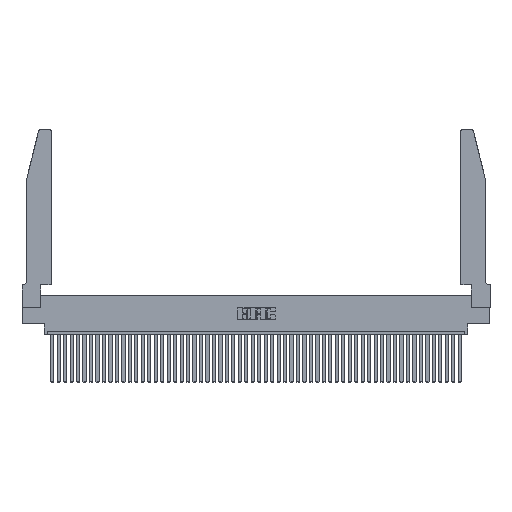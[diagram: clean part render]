
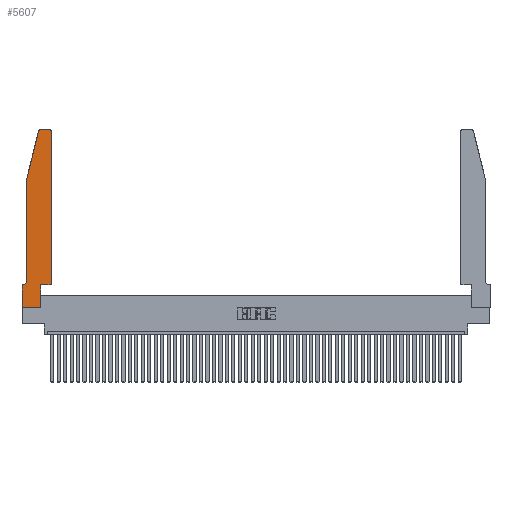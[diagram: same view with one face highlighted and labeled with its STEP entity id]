
A CAD part, top view. The second image highlights one B-rep face of the part: STEP entity #5607.
In plain terms, the highlighted planar face has unit normal (0, 0, 1).
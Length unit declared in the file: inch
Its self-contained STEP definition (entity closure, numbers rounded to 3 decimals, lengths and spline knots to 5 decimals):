
#176 = LINE ( 'NONE', #29525, #39927 ) ;
#770 = EDGE_CURVE ( 'NONE', #45909, #34590, #813, .T. ) ;
#813 = CIRCLE ( 'NONE', #7433, 0.03 ) ;
#827 = DIRECTION ( 'NONE',  ( 0., -1., 0. ) ) ;
#975 = DIRECTION ( 'NONE',  ( 0., 0., -1. ) ) ;
#992 = EDGE_CURVE ( 'NONE', #42682, #34674, #176, .T. ) ;
#1034 = DIRECTION ( 'NONE',  ( 0., 1., 0. ) ) ;
#1082 = LINE ( 'NONE', #16344, #42033 ) ;
#1908 = CARTESIAN_POINT ( 'NONE',  ( 0.284, 2.75, 0.37 ) ) ;
#1987 = VERTEX_POINT ( 'NONE', #20267 ) ;
#2235 = EDGE_CURVE ( 'NONE', #44550, #41243, #7858, .T. ) ;
#3625 = EDGE_CURVE ( 'NONE', #34590, #21164, #1082, .T. ) ;
#3670 = CARTESIAN_POINT ( 'NONE',  ( 0.4505, 0.35, 0.37 ) ) ;
#4060 = VECTOR ( 'NONE', #827, 39.37008 ) ;
#4079 = CARTESIAN_POINT ( 'NONE',  ( 0.4205, 2.75, 0.37 ) ) ;
#4171 = ORIENTED_EDGE ( 'NONE', *, *, #770, .T. ) ;
#5479 = ORIENTED_EDGE ( 'NONE', *, *, #24863, .T. ) ;
#5539 = CARTESIAN_POINT ( 'NONE',  ( 0.2605, 2.75, 0.37 ) ) ;
#5607 = ADVANCED_FACE ( 'NONE', ( #14952 ), #9008, .T. ) ;
#6167 = EDGE_CURVE ( 'NONE', #41243, #20302, #34780, .T. ) ;
#7433 = AXIS2_PLACEMENT_3D ( 'NONE', #32642, #35821, #12720 ) ;
#7858 = LINE ( 'NONE', #30614, #26554 ) ;
#8378 = EDGE_CURVE ( 'NONE', #34674, #22963, #16370, .T. ) ;
#8766 = DIRECTION ( 'NONE',  ( -0.239, -0.971, 0. ) ) ;
#9008 = PLANE ( 'NONE',  #36637 ) ;
#10005 = CARTESIAN_POINT ( 'NONE',  ( 0.4505, 0.35, 0.37 ) ) ;
#11383 = VECTOR ( 'NONE', #28150, 39.37008 ) ;
#11544 = EDGE_CURVE ( 'NONE', #1987, #44550, #13469, .T. ) ;
#12720 = DIRECTION ( 'NONE',  ( 1., 0., 0. ) ) ;
#13128 = VERTEX_POINT ( 'NONE', #47559 ) ;
#13206 = ORIENTED_EDGE ( 'NONE', *, *, #48913, .T. ) ;
#13469 = LINE ( 'NONE', #34265, #43015 ) ;
#13488 = CARTESIAN_POINT ( 'NONE',  ( 0.2865, 0., 0.37 ) ) ;
#14952 = FACE_OUTER_BOUND ( 'NONE', #37330, .T. ) ;
#16344 = CARTESIAN_POINT ( 'NONE',  ( 0.0755, 2., 0.37 ) ) ;
#16370 = CIRCLE ( 'NONE', #36065, 0.03 ) ;
#17227 = VECTOR ( 'NONE', #30467, 39.37008 ) ;
#18933 = CARTESIAN_POINT ( 'NONE',  ( 0.0055, 0.42, 0.37 ) ) ;
#19455 = CARTESIAN_POINT ( 'NONE',  ( 0.0755, 2., 0.37 ) ) ;
#19978 = DIRECTION ( 'NONE',  ( 0., 0., 1. ) ) ;
#20267 = CARTESIAN_POINT ( 'NONE',  ( 0.0055, 0.35, 0.37 ) ) ;
#20302 = VERTEX_POINT ( 'NONE', #13488 ) ;
#20614 = ORIENTED_EDGE ( 'NONE', *, *, #36478, .T. ) ;
#20902 = LINE ( 'NONE', #47099, #4060 ) ;
#21164 = VERTEX_POINT ( 'NONE', #19455 ) ;
#21502 = CARTESIAN_POINT ( 'NONE',  ( 0.4505, 2.72, 0.37 ) ) ;
#22963 = VERTEX_POINT ( 'NONE', #4079 ) ;
#23854 = DIRECTION ( 'NONE',  ( -1., 0., 0. ) ) ;
#23931 = ORIENTED_EDGE ( 'NONE', *, *, #8378, .T. ) ;
#24050 = AXIS2_PLACEMENT_3D ( 'NONE', #18933, #975, #23854 ) ;
#24863 = EDGE_CURVE ( 'NONE', #22963, #45909, #40919, .T. ) ;
#25529 = CARTESIAN_POINT ( 'NONE',  ( 0., 0., 0.37 ) ) ;
#26346 = EDGE_CURVE ( 'NONE', #20302, #43170, #49282, .T. ) ;
#26402 = DIRECTION ( 'NONE',  ( 1., 0., 0. ) ) ;
#26513 = DIRECTION ( 'NONE',  ( -1., 0., 0. ) ) ;
#26554 = VECTOR ( 'NONE', #34469, 39.37008 ) ;
#27685 = VECTOR ( 'NONE', #36986, 39.37008 ) ;
#27927 = CARTESIAN_POINT ( 'NONE',  ( 0., 0.35, 0.37 ) ) ;
#28104 = ORIENTED_EDGE ( 'NONE', *, *, #6167, .T. ) ;
#28150 = DIRECTION ( 'NONE',  ( -1., 0., 0. ) ) ;
#29525 = CARTESIAN_POINT ( 'NONE',  ( 0.4505, 0.35, 0.37 ) ) ;
#30467 = DIRECTION ( 'NONE',  ( 1., 0., 0. ) ) ;
#30614 = CARTESIAN_POINT ( 'NONE',  ( 0., 0., 0.37 ) ) ;
#31901 = CARTESIAN_POINT ( 'NONE',  ( 0., 0.35, 0.37 ) ) ;
#32642 = CARTESIAN_POINT ( 'NONE',  ( 0.284, 2.72, 0.37 ) ) ;
#34265 = CARTESIAN_POINT ( 'NONE',  ( 0.0755, 0.35, 0.37 ) ) ;
#34469 = DIRECTION ( 'NONE',  ( 0., -1., 0. ) ) ;
#34531 = EDGE_CURVE ( 'NONE', #21164, #13128, #20902, .T. ) ;
#34535 = CARTESIAN_POINT ( 'NONE',  ( 0.2865, 0.35, 0.37 ) ) ;
#34590 = VERTEX_POINT ( 'NONE', #47611 ) ;
#34674 = VERTEX_POINT ( 'NONE', #21502 ) ;
#34780 = LINE ( 'NONE', #42061, #17227 ) ;
#35309 = ORIENTED_EDGE ( 'NONE', *, *, #26346, .T. ) ;
#35821 = DIRECTION ( 'NONE',  ( 0., 0., 1. ) ) ;
#35978 = DIRECTION ( 'NONE',  ( 1., 0., 0. ) ) ;
#36065 = AXIS2_PLACEMENT_3D ( 'NONE', #43526, #44383, #26402 ) ;
#36478 = EDGE_CURVE ( 'NONE', #43170, #42682, #36683, .T. ) ;
#36637 = AXIS2_PLACEMENT_3D ( 'NONE', #27927, #19978, #35978 ) ;
#36657 = CARTESIAN_POINT ( 'NONE',  ( 0.2865, 0.35, 0.37 ) ) ;
#36683 = LINE ( 'NONE', #10005, #27685 ) ;
#36986 = DIRECTION ( 'NONE',  ( 1., 0., 0. ) ) ;
#37330 = EDGE_LOOP ( 'NONE', ( #5479, #4171, #47223, #47231, #13206, #38351, #49577, #28104, #35309, #20614, #37728, #23931 ) ) ;
#37728 = ORIENTED_EDGE ( 'NONE', *, *, #992, .T. ) ;
#38351 = ORIENTED_EDGE ( 'NONE', *, *, #11544, .T. ) ;
#38995 = VECTOR ( 'NONE', #44572, 39.37008 ) ;
#39927 = VECTOR ( 'NONE', #1034, 39.37008 ) ;
#40919 = LINE ( 'NONE', #5539, #11383 ) ;
#41243 = VERTEX_POINT ( 'NONE', #25529 ) ;
#42033 = VECTOR ( 'NONE', #8766, 39.37008 ) ;
#42061 = CARTESIAN_POINT ( 'NONE',  ( 0., 0., 0.37 ) ) ;
#42682 = VERTEX_POINT ( 'NONE', #3670 ) ;
#43015 = VECTOR ( 'NONE', #26513, 39.37008 ) ;
#43170 = VERTEX_POINT ( 'NONE', #34535 ) ;
#43526 = CARTESIAN_POINT ( 'NONE',  ( 0.4205, 2.72, 0.37 ) ) ;
#44383 = DIRECTION ( 'NONE',  ( 0., 0., 1. ) ) ;
#44550 = VERTEX_POINT ( 'NONE', #31901 ) ;
#44572 = DIRECTION ( 'NONE',  ( 0., 1., 0. ) ) ;
#45543 = CIRCLE ( 'NONE', #24050, 0.07 ) ;
#45909 = VERTEX_POINT ( 'NONE', #1908 ) ;
#47099 = CARTESIAN_POINT ( 'NONE',  ( 0.0755, 2., 0.37 ) ) ;
#47223 = ORIENTED_EDGE ( 'NONE', *, *, #3625, .T. ) ;
#47231 = ORIENTED_EDGE ( 'NONE', *, *, #34531, .T. ) ;
#47559 = CARTESIAN_POINT ( 'NONE',  ( 0.0755, 0.42, 0.37 ) ) ;
#47611 = CARTESIAN_POINT ( 'NONE',  ( 0.25487, 2.72718, 0.37 ) ) ;
#48913 = EDGE_CURVE ( 'NONE', #13128, #1987, #45543, .T. ) ;
#49282 = LINE ( 'NONE', #36657, #38995 ) ;
#49577 = ORIENTED_EDGE ( 'NONE', *, *, #2235, .T. ) ;
